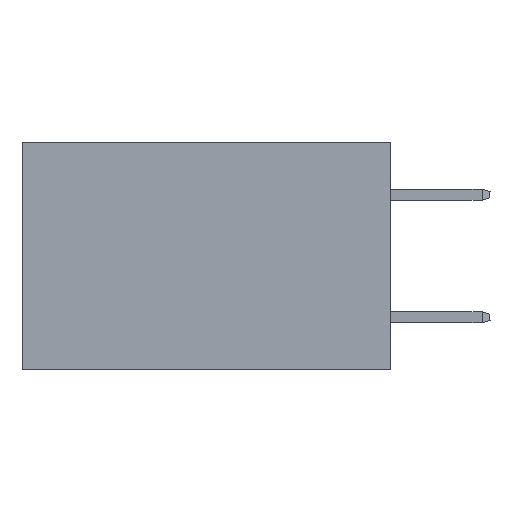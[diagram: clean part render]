
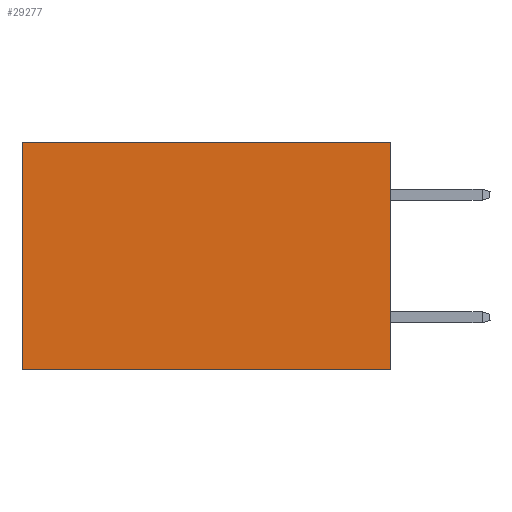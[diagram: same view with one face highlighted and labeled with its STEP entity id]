
A CAD part, left-side view. The second image highlights one B-rep face of the part: STEP entity #29277.
In plain terms, the highlighted planar face has unit normal (-1, 0, 0).
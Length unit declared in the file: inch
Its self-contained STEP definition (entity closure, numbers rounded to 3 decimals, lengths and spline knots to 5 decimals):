
#2755 = VERTEX_POINT ( 'NONE', #41013 ) ;
#5005 = AXIS2_PLACEMENT_3D ( 'NONE', #6076, #9609, #16610 ) ;
#6076 = CARTESIAN_POINT ( 'NONE',  ( 0.2875, 0., 0. ) ) ;
#6906 = CARTESIAN_POINT ( 'NONE',  ( 0.2875, 0., -0.37 ) ) ;
#9020 = PLANE ( 'NONE',  #5005 ) ;
#9373 = DIRECTION ( 'NONE',  ( 0., 1., 0. ) ) ;
#9609 = DIRECTION ( 'NONE',  ( 1., 0., 0. ) ) ;
#11511 = VERTEX_POINT ( 'NONE', #32078 ) ;
#12890 = VERTEX_POINT ( 'NONE', #39955 ) ;
#15528 = VECTOR ( 'NONE', #27929, 39.37008 ) ;
#16180 = EDGE_LOOP ( 'NONE', ( #24563, #37524, #33873, #35692 ) ) ;
#16463 = EDGE_CURVE ( 'NONE', #2755, #12890, #45016, .T. ) ;
#16610 = DIRECTION ( 'NONE',  ( 0., 0., -1. ) ) ;
#17239 = EDGE_CURVE ( 'NONE', #12890, #28226, #26979, .T. ) ;
#18043 = CARTESIAN_POINT ( 'NONE',  ( 0.2875, 0.6, -0.37 ) ) ;
#19636 = DIRECTION ( 'NONE',  ( 0., 0., -1. ) ) ;
#19788 = CARTESIAN_POINT ( 'NONE',  ( 0.2875, 0., 0. ) ) ;
#22700 = VECTOR ( 'NONE', #19636, 39.37008 ) ;
#24563 = ORIENTED_EDGE ( 'NONE', *, *, #34767, .T. ) ;
#25500 = CARTESIAN_POINT ( 'NONE',  ( 0.2875, 0.6, 0. ) ) ;
#25798 = DIRECTION ( 'NONE',  ( 0., 0., -1. ) ) ;
#26163 = FACE_OUTER_BOUND ( 'NONE', #16180, .T. ) ;
#26979 = LINE ( 'NONE', #6906, #15528 ) ;
#27929 = DIRECTION ( 'NONE',  ( 0., 1., 0. ) ) ;
#28226 = VERTEX_POINT ( 'NONE', #18043 ) ;
#28600 = EDGE_CURVE ( 'NONE', #2755, #11511, #29401, .T. ) ;
#29277 = ADVANCED_FACE ( 'NONE', ( #26163 ), #9020, .F. ) ;
#29401 = LINE ( 'NONE', #33286, #44658 ) ;
#30296 = LINE ( 'NONE', #25500, #38467 ) ;
#32078 = CARTESIAN_POINT ( 'NONE',  ( 0.2875, 0.6, 0. ) ) ;
#33286 = CARTESIAN_POINT ( 'NONE',  ( 0.2875, 0., 0. ) ) ;
#33873 = ORIENTED_EDGE ( 'NONE', *, *, #16463, .F. ) ;
#34767 = EDGE_CURVE ( 'NONE', #11511, #28226, #30296, .T. ) ;
#35692 = ORIENTED_EDGE ( 'NONE', *, *, #28600, .T. ) ;
#37524 = ORIENTED_EDGE ( 'NONE', *, *, #17239, .F. ) ;
#38467 = VECTOR ( 'NONE', #25798, 39.37008 ) ;
#39955 = CARTESIAN_POINT ( 'NONE',  ( 0.2875, 0., -0.37 ) ) ;
#41013 = CARTESIAN_POINT ( 'NONE',  ( 0.2875, 0., 0. ) ) ;
#44658 = VECTOR ( 'NONE', #9373, 39.37008 ) ;
#45016 = LINE ( 'NONE', #19788, #22700 ) ;
